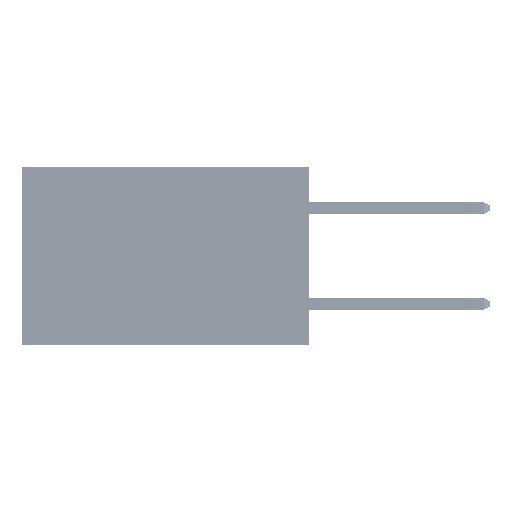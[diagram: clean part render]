
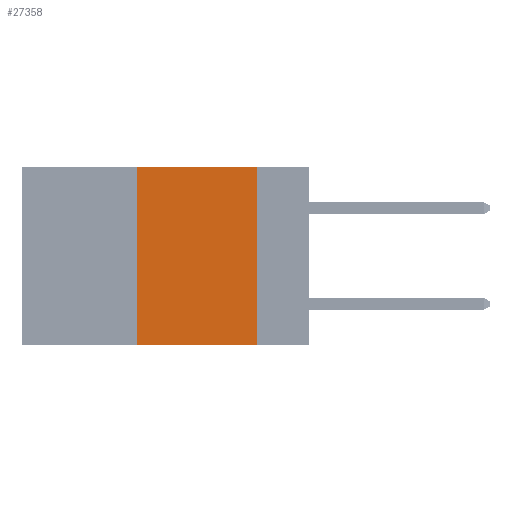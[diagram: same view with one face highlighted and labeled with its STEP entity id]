
A CAD part, left-side view. The second image highlights one B-rep face of the part: STEP entity #27358.
In plain terms, the highlighted planar face has unit normal (-1, 0, 0).
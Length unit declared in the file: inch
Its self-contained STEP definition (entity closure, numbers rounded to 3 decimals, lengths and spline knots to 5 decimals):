
#1111 = EDGE_CURVE ( 'NONE', #32068, #23661, #30732, .T. ) ;
#2192 = LINE ( 'NONE', #50772, #10738 ) ;
#2339 = CARTESIAN_POINT ( 'NONE',  ( 0., 0.6, 0. ) ) ;
#2579 = CARTESIAN_POINT ( 'NONE',  ( 0., 0.11, 0. ) ) ;
#3777 = VERTEX_POINT ( 'NONE', #30921 ) ;
#7875 = EDGE_CURVE ( 'NONE', #17229, #23661, #52117, .T. ) ;
#7968 = VECTOR ( 'NONE', #27489, 39.37008 ) ;
#9740 = LINE ( 'NONE', #2339, #52220 ) ;
#10738 = VECTOR ( 'NONE', #14641, 39.37008 ) ;
#11089 = EDGE_CURVE ( 'NONE', #17229, #3777, #2192, .T. ) ;
#11763 = DIRECTION ( 'NONE',  ( 0., -1., 0. ) ) ;
#13111 = CARTESIAN_POINT ( 'NONE',  ( 0., 0.11, -0.37 ) ) ;
#14456 = CARTESIAN_POINT ( 'NONE',  ( 0., 0.36, -0.37 ) ) ;
#14641 = DIRECTION ( 'NONE',  ( 0., 0., 1. ) ) ;
#15766 = CARTESIAN_POINT ( 'NONE',  ( 0., 0.6, -0.37 ) ) ;
#16986 = CARTESIAN_POINT ( 'NONE',  ( 0., 0.6, 0. ) ) ;
#17229 = VERTEX_POINT ( 'NONE', #14456 ) ;
#23661 = VERTEX_POINT ( 'NONE', #13111 ) ;
#24937 = FACE_OUTER_BOUND ( 'NONE', #33484, .T. ) ;
#25991 = DIRECTION ( 'NONE',  ( 0., 0., -1. ) ) ;
#26898 = ORIENTED_EDGE ( 'NONE', *, *, #11089, .F. ) ;
#27358 = ADVANCED_FACE ( 'NONE', ( #24937 ), #50416, .F. ) ;
#27489 = DIRECTION ( 'NONE',  ( 0., 0., -1. ) ) ;
#29025 = EDGE_CURVE ( 'NONE', #3777, #32068, #9740, .T. ) ;
#30436 = ORIENTED_EDGE ( 'NONE', *, *, #29025, .F. ) ;
#30732 = LINE ( 'NONE', #2579, #7968 ) ;
#30921 = CARTESIAN_POINT ( 'NONE',  ( 0., 0.36, 0. ) ) ;
#32068 = VERTEX_POINT ( 'NONE', #34191 ) ;
#33484 = EDGE_LOOP ( 'NONE', ( #47253, #30436, #26898, #37232 ) ) ;
#34191 = CARTESIAN_POINT ( 'NONE',  ( 0., 0.11, 0. ) ) ;
#35176 = AXIS2_PLACEMENT_3D ( 'NONE', #16986, #49891, #25991 ) ;
#37232 = ORIENTED_EDGE ( 'NONE', *, *, #7875, .T. ) ;
#41287 = VECTOR ( 'NONE', #11763, 39.37008 ) ;
#46090 = DIRECTION ( 'NONE',  ( 0., -1., 0. ) ) ;
#47253 = ORIENTED_EDGE ( 'NONE', *, *, #1111, .F. ) ;
#49891 = DIRECTION ( 'NONE',  ( 1., 0., 0. ) ) ;
#50416 = PLANE ( 'NONE',  #35176 ) ;
#50772 = CARTESIAN_POINT ( 'NONE',  ( 0., 0.36, 0. ) ) ;
#52117 = LINE ( 'NONE', #15766, #41287 ) ;
#52220 = VECTOR ( 'NONE', #46090, 39.37008 ) ;
